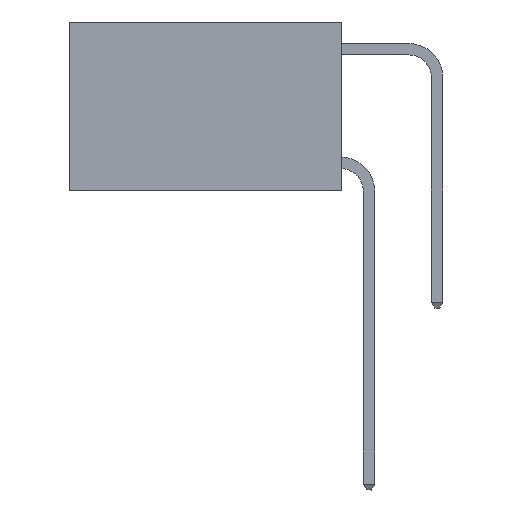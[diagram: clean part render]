
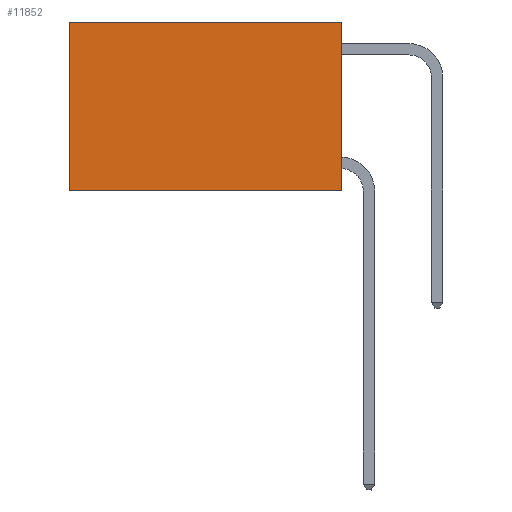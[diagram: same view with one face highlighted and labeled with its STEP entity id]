
A CAD part, left-side view. The second image highlights one B-rep face of the part: STEP entity #11852.
In plain terms, the highlighted planar face has unit normal (-1, 0, 0).
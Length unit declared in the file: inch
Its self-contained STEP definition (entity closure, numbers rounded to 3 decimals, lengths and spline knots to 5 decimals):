
#795 = ORIENTED_EDGE ( 'NONE', *, *, #1377, .T. ) ;
#996 = ORIENTED_EDGE ( 'NONE', *, *, #25404, .F. ) ;
#1377 = EDGE_CURVE ( 'NONE', #12426, #11732, #15203, .T. ) ;
#1788 = VERTEX_POINT ( 'NONE', #13802 ) ;
#2170 = EDGE_CURVE ( 'NONE', #1788, #2331, #18368, .T. ) ;
#2331 = VERTEX_POINT ( 'NONE', #23015 ) ;
#2350 = DIRECTION ( 'NONE',  ( 0., 0., -1. ) ) ;
#3683 = LINE ( 'NONE', #21856, #23988 ) ;
#6392 = PLANE ( 'NONE',  #29463 ) ;
#10445 = CARTESIAN_POINT ( 'NONE',  ( 0.2625, 0.6, 0. ) ) ;
#10971 = CARTESIAN_POINT ( 'NONE',  ( 0.2625, 0., 0. ) ) ;
#11106 = FACE_OUTER_BOUND ( 'NONE', #13414, .T. ) ;
#11732 = VERTEX_POINT ( 'NONE', #23840 ) ;
#11852 = ADVANCED_FACE ( 'NONE', ( #11106 ), #6392, .F. ) ;
#12426 = VERTEX_POINT ( 'NONE', #10445 ) ;
#12713 = DIRECTION ( 'NONE',  ( 1., 0., 0. ) ) ;
#13191 = LINE ( 'NONE', #22036, #14933 ) ;
#13414 = EDGE_LOOP ( 'NONE', ( #795, #996, #27941, #25480 ) ) ;
#13441 = VECTOR ( 'NONE', #2350, 39.37008 ) ;
#13802 = CARTESIAN_POINT ( 'NONE',  ( 0.2625, 0., 0. ) ) ;
#14933 = VECTOR ( 'NONE', #17513, 39.37008 ) ;
#15203 = LINE ( 'NONE', #22573, #13441 ) ;
#15629 = DIRECTION ( 'NONE',  ( 0., 1., 0. ) ) ;
#17313 = DIRECTION ( 'NONE',  ( 0., 0., -1. ) ) ;
#17513 = DIRECTION ( 'NONE',  ( 0., 1., 0. ) ) ;
#18368 = LINE ( 'NONE', #28739, #21255 ) ;
#21255 = VECTOR ( 'NONE', #22231, 39.37008 ) ;
#21856 = CARTESIAN_POINT ( 'NONE',  ( 0.2625, 0., 0. ) ) ;
#22036 = CARTESIAN_POINT ( 'NONE',  ( 0.2625, 0., -0.37 ) ) ;
#22231 = DIRECTION ( 'NONE',  ( 0., 0., -1. ) ) ;
#22573 = CARTESIAN_POINT ( 'NONE',  ( 0.2625, 0.6, 0. ) ) ;
#23015 = CARTESIAN_POINT ( 'NONE',  ( 0.2625, 0., -0.37 ) ) ;
#23771 = EDGE_CURVE ( 'NONE', #1788, #12426, #3683, .T. ) ;
#23840 = CARTESIAN_POINT ( 'NONE',  ( 0.2625, 0.6, -0.37 ) ) ;
#23988 = VECTOR ( 'NONE', #15629, 39.37008 ) ;
#25404 = EDGE_CURVE ( 'NONE', #2331, #11732, #13191, .T. ) ;
#25480 = ORIENTED_EDGE ( 'NONE', *, *, #23771, .T. ) ;
#27941 = ORIENTED_EDGE ( 'NONE', *, *, #2170, .F. ) ;
#28739 = CARTESIAN_POINT ( 'NONE',  ( 0.2625, 0., 0. ) ) ;
#29463 = AXIS2_PLACEMENT_3D ( 'NONE', #10971, #12713, #17313 ) ;
